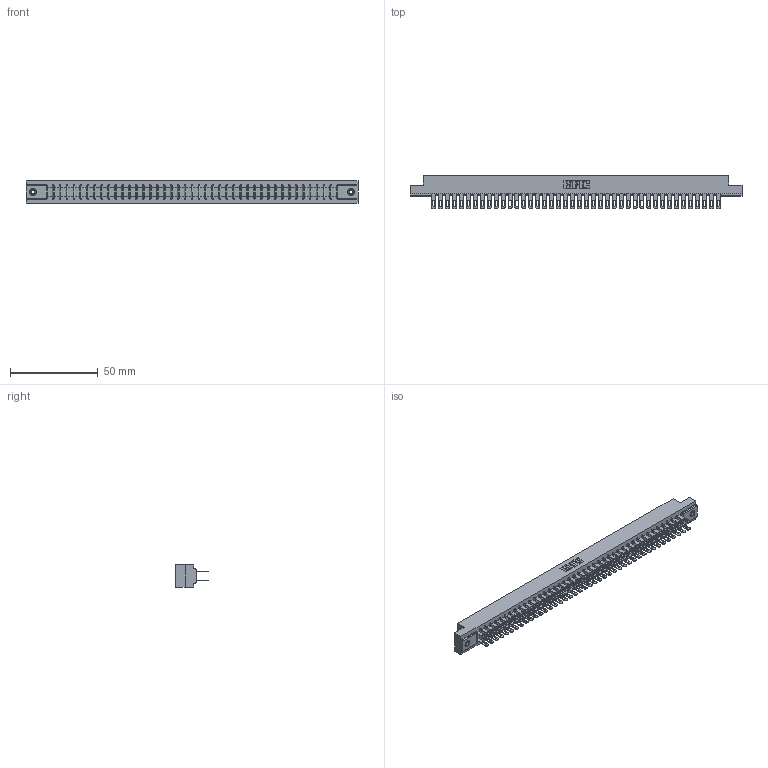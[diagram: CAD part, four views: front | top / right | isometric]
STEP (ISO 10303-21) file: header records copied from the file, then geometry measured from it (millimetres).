
FILE_DESCRIPTION (( 'STEP AP203' ), '1' );
FILE_NAME ('357-084-500-208.STEP', '2019-09-19T17:29:54', ( '' ), ( '' ), 'SwSTEP 2.0', 'SolidWorks 2016', '' );
FILE_SCHEMA (( 'CONFIG_CONTROL_DESIGN' ));
Length unit declared in the file: inch
Products named in the file (4): 307 Part_.156 Dia Mounting Holes; 345-250-001_345-250-003-102; 357-084-500-208; 307-290-001_500
Assembly tree (87 placements, depth 2):
  357-084-500-208
    307 Part_.156 Dia Mounting Holes
    307-290-001_500  x84
    345-250-001_345-250-003-102  x2
Bounding box: 189.43 x 19.18 x 12.7 mm (x, y, z)
Volume: 20378.2 mm3; surface area: 26291.3 mm2
Topology: 87 solids, 87 shells, 4085 faces, 11379 edges, 7350 vertices
Faces by surface type: plane 2622, cylinder 1361, sphere 86, cone 12, torus 4
Entity records: 38509 total; most frequent: CARTESIAN_POINT 6281, ORIENTED_EDGE 6218, DIRECTION 6163, EDGE_CURVE 3109, LINE 2383, VECTOR 2383, VERTEX_POINT 2008, AXIS2_PLACEMENT_3D 1890
